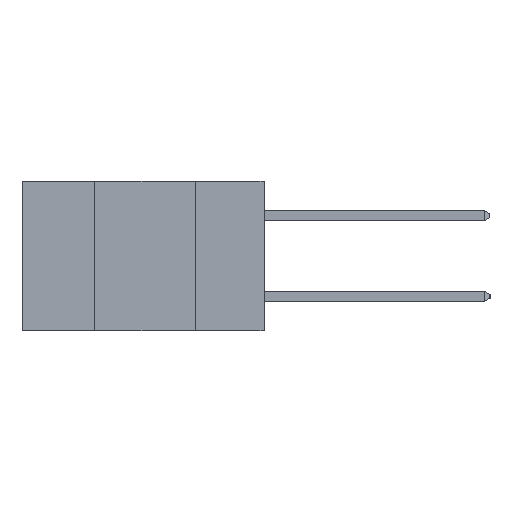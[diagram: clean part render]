
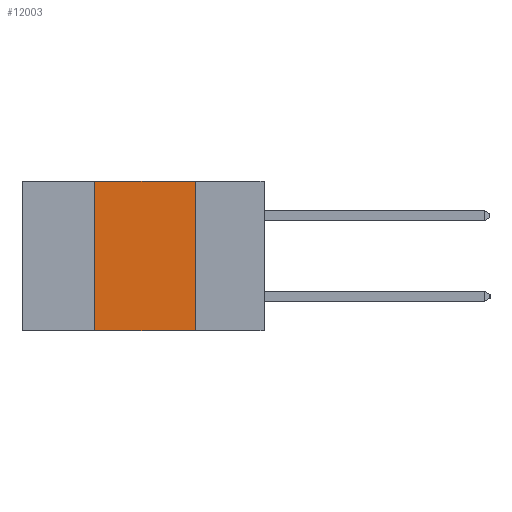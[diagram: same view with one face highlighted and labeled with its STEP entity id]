
A CAD part, left-side view. The second image highlights one B-rep face of the part: STEP entity #12003.
In plain terms, the highlighted planar face has unit normal (-1, 0, 0).
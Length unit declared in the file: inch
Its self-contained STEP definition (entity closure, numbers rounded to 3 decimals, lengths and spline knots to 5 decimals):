
#688 = CARTESIAN_POINT ( 'NONE',  ( 0., 0.42, 0. ) ) ;
#770 = EDGE_CURVE ( 'NONE', #6934, #12919, #10285, .T. ) ;
#1271 = PLANE ( 'NONE',  #2169 ) ;
#1598 = EDGE_LOOP ( 'NONE', ( #13561, #1818, #14087, #13582 ) ) ;
#1818 = ORIENTED_EDGE ( 'NONE', *, *, #770, .F. ) ;
#1864 = EDGE_CURVE ( 'NONE', #3334, #6934, #19342, .T. ) ;
#1940 = CARTESIAN_POINT ( 'NONE',  ( 0., 0.42, -0.37 ) ) ;
#1976 = DIRECTION ( 'NONE',  ( 0., 0., -1. ) ) ;
#2169 = AXIS2_PLACEMENT_3D ( 'NONE', #12463, #2883, #14089 ) ;
#2428 = CARTESIAN_POINT ( 'NONE',  ( 0., 0.42, -0.37 ) ) ;
#2883 = DIRECTION ( 'NONE',  ( 1., 0., 0. ) ) ;
#2957 = LINE ( 'NONE', #8140, #19321 ) ;
#3334 = VERTEX_POINT ( 'NONE', #2428 ) ;
#3559 = CARTESIAN_POINT ( 'NONE',  ( 0., 0.17, 0. ) ) ;
#6934 = VERTEX_POINT ( 'NONE', #688 ) ;
#7793 = LINE ( 'NONE', #11524, #15765 ) ;
#8140 = CARTESIAN_POINT ( 'NONE',  ( 0., 0.6, -0.37 ) ) ;
#9753 = DIRECTION ( 'NONE',  ( 0., -1., 0. ) ) ;
#10285 = LINE ( 'NONE', #17106, #14563 ) ;
#11269 = DIRECTION ( 'NONE',  ( 0., 0., 1. ) ) ;
#11477 = EDGE_CURVE ( 'NONE', #3334, #13628, #2957, .T. ) ;
#11524 = CARTESIAN_POINT ( 'NONE',  ( 0., 0.17, -0.37 ) ) ;
#12003 = ADVANCED_FACE ( 'NONE', ( #18343 ), #1271, .F. ) ;
#12463 = CARTESIAN_POINT ( 'NONE',  ( 0., 0.6, 0. ) ) ;
#12919 = VERTEX_POINT ( 'NONE', #3559 ) ;
#13561 = ORIENTED_EDGE ( 'NONE', *, *, #18237, .F. ) ;
#13582 = ORIENTED_EDGE ( 'NONE', *, *, #11477, .T. ) ;
#13628 = VERTEX_POINT ( 'NONE', #17155 ) ;
#14087 = ORIENTED_EDGE ( 'NONE', *, *, #1864, .F. ) ;
#14089 = DIRECTION ( 'NONE',  ( 0., 0., -1. ) ) ;
#14563 = VECTOR ( 'NONE', #16557, 39.37008 ) ;
#15231 = VECTOR ( 'NONE', #11269, 39.37008 ) ;
#15765 = VECTOR ( 'NONE', #1976, 39.37008 ) ;
#16557 = DIRECTION ( 'NONE',  ( 0., -1., 0. ) ) ;
#17106 = CARTESIAN_POINT ( 'NONE',  ( 0., 0.6, 0. ) ) ;
#17155 = CARTESIAN_POINT ( 'NONE',  ( 0., 0.17, -0.37 ) ) ;
#18237 = EDGE_CURVE ( 'NONE', #12919, #13628, #7793, .T. ) ;
#18343 = FACE_OUTER_BOUND ( 'NONE', #1598, .T. ) ;
#19321 = VECTOR ( 'NONE', #9753, 39.37008 ) ;
#19342 = LINE ( 'NONE', #1940, #15231 ) ;
